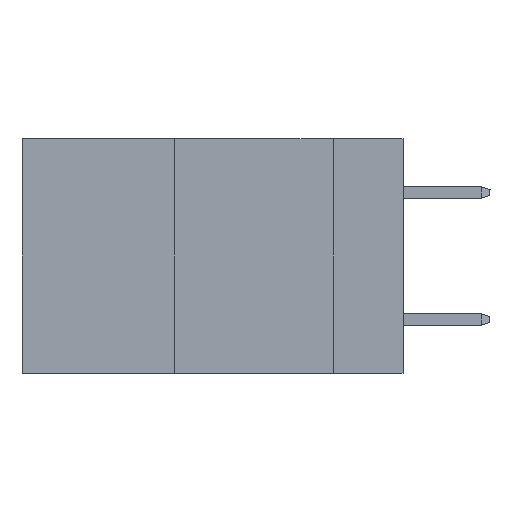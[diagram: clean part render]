
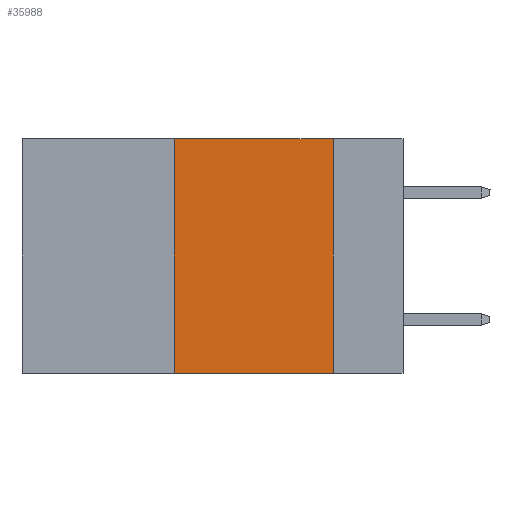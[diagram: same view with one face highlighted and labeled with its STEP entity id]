
A CAD part, left-side view. The second image highlights one B-rep face of the part: STEP entity #35988.
In plain terms, the highlighted planar face has unit normal (-1, 0, 0).
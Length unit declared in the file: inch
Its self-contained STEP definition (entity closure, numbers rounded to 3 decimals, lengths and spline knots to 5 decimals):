
#190 = ORIENTED_EDGE ( 'NONE', *, *, #5853, .F. ) ;
#2192 = AXIS2_PLACEMENT_3D ( 'NONE', #11023, #41149, #4840 ) ;
#3898 = ORIENTED_EDGE ( 'NONE', *, *, #14573, .T. ) ;
#4442 = VECTOR ( 'NONE', #25471, 39.37008 ) ;
#4840 = DIRECTION ( 'NONE',  ( 0., 0., -1. ) ) ;
#4891 = CARTESIAN_POINT ( 'NONE',  ( 0., 0.11, -0.37 ) ) ;
#5062 = VECTOR ( 'NONE', #8592, 39.37008 ) ;
#5853 = EDGE_CURVE ( 'NONE', #13867, #16435, #18636, .T. ) ;
#8592 = DIRECTION ( 'NONE',  ( 0., 0., 1. ) ) ;
#9695 = CARTESIAN_POINT ( 'NONE',  ( 0., 0.6, -0.37 ) ) ;
#11023 = CARTESIAN_POINT ( 'NONE',  ( 0., 0.6, 0. ) ) ;
#11651 = DIRECTION ( 'NONE',  ( 0., -1., 0. ) ) ;
#13867 = VERTEX_POINT ( 'NONE', #14454 ) ;
#14217 = FACE_OUTER_BOUND ( 'NONE', #16690, .T. ) ;
#14454 = CARTESIAN_POINT ( 'NONE',  ( 0., 0.36, -0.37 ) ) ;
#14573 = EDGE_CURVE ( 'NONE', #13867, #27459, #38976, .T. ) ;
#16435 = VERTEX_POINT ( 'NONE', #30536 ) ;
#16690 = EDGE_LOOP ( 'NONE', ( #40262, #40591, #190, #3898 ) ) ;
#18636 = LINE ( 'NONE', #37896, #5062 ) ;
#19804 = PLANE ( 'NONE',  #2192 ) ;
#20831 = CARTESIAN_POINT ( 'NONE',  ( 0., 0.11, 0. ) ) ;
#22730 = DIRECTION ( 'NONE',  ( 0., -1., 0. ) ) ;
#24782 = VECTOR ( 'NONE', #22730, 39.37008 ) ;
#25047 = LINE ( 'NONE', #41898, #4442 ) ;
#25471 = DIRECTION ( 'NONE',  ( 0., 0., -1. ) ) ;
#26811 = EDGE_CURVE ( 'NONE', #16435, #38096, #31783, .T. ) ;
#27459 = VERTEX_POINT ( 'NONE', #4891 ) ;
#28987 = CARTESIAN_POINT ( 'NONE',  ( 0., 0.6, 0. ) ) ;
#30536 = CARTESIAN_POINT ( 'NONE',  ( 0., 0.36, 0. ) ) ;
#31783 = LINE ( 'NONE', #28987, #40330 ) ;
#35988 = ADVANCED_FACE ( 'NONE', ( #14217 ), #19804, .F. ) ;
#37896 = CARTESIAN_POINT ( 'NONE',  ( 0., 0.36, 0. ) ) ;
#38096 = VERTEX_POINT ( 'NONE', #20831 ) ;
#38976 = LINE ( 'NONE', #9695, #24782 ) ;
#40262 = ORIENTED_EDGE ( 'NONE', *, *, #40379, .F. ) ;
#40330 = VECTOR ( 'NONE', #11651, 39.37008 ) ;
#40379 = EDGE_CURVE ( 'NONE', #38096, #27459, #25047, .T. ) ;
#40591 = ORIENTED_EDGE ( 'NONE', *, *, #26811, .F. ) ;
#41149 = DIRECTION ( 'NONE',  ( 1., 0., 0. ) ) ;
#41898 = CARTESIAN_POINT ( 'NONE',  ( 0., 0.11, 0. ) ) ;
